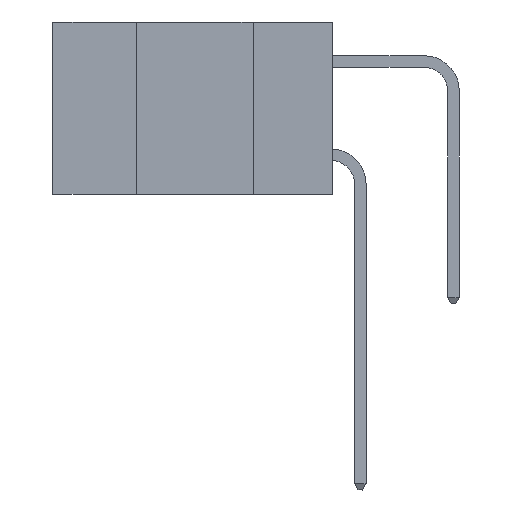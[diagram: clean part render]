
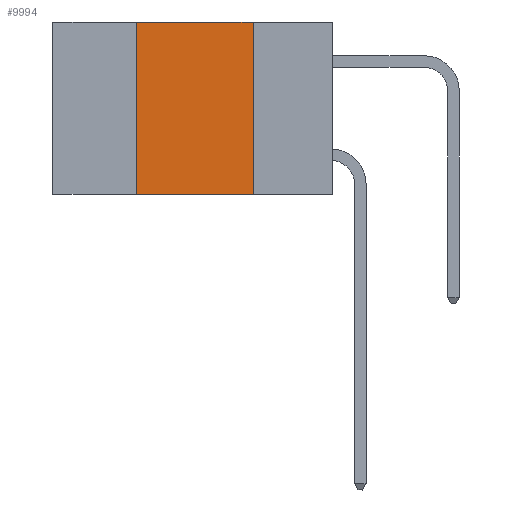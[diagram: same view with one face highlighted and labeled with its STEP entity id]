
A CAD part, left-side view. The second image highlights one B-rep face of the part: STEP entity #9994.
In plain terms, the highlighted planar face has unit normal (-1, 0, 0).
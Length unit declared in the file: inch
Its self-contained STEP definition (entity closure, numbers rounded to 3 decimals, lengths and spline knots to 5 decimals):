
#310 = CARTESIAN_POINT ( 'NONE',  ( 0., 0.42, 0. ) ) ;
#703 = FACE_OUTER_BOUND ( 'NONE', #6373, .T. ) ;
#1762 = LINE ( 'NONE', #10228, #7416 ) ;
#2990 = ORIENTED_EDGE ( 'NONE', *, *, #6395, .F. ) ;
#3064 = CARTESIAN_POINT ( 'NONE',  ( 0., 0.17, 0. ) ) ;
#3748 = LINE ( 'NONE', #3064, #11053 ) ;
#3896 = VERTEX_POINT ( 'NONE', #12928 ) ;
#4697 = DIRECTION ( 'NONE',  ( 0., 0., -1. ) ) ;
#4944 = VECTOR ( 'NONE', #11201, 39.37008 ) ;
#5253 = CARTESIAN_POINT ( 'NONE',  ( 0., 0.42, 0. ) ) ;
#5281 = DIRECTION ( 'NONE',  ( 0., -1., 0. ) ) ;
#5345 = CARTESIAN_POINT ( 'NONE',  ( 0., 0.6, 0. ) ) ;
#5495 = VERTEX_POINT ( 'NONE', #11802 ) ;
#6373 = EDGE_LOOP ( 'NONE', ( #9705, #7972, #2990, #8277 ) ) ;
#6395 = EDGE_CURVE ( 'NONE', #7828, #7204, #9927, .T. ) ;
#7115 = EDGE_CURVE ( 'NONE', #7828, #5495, #1762, .T. ) ;
#7204 = VERTEX_POINT ( 'NONE', #310 ) ;
#7416 = VECTOR ( 'NONE', #5281, 39.37008 ) ;
#7660 = CARTESIAN_POINT ( 'NONE',  ( 0., 0.6, 0. ) ) ;
#7828 = VERTEX_POINT ( 'NONE', #12256 ) ;
#7972 = ORIENTED_EDGE ( 'NONE', *, *, #8352, .F. ) ;
#8277 = ORIENTED_EDGE ( 'NONE', *, *, #7115, .T. ) ;
#8352 = EDGE_CURVE ( 'NONE', #7204, #3896, #9423, .T. ) ;
#9032 = DIRECTION ( 'NONE',  ( 0., 0., -1. ) ) ;
#9303 = AXIS2_PLACEMENT_3D ( 'NONE', #7660, #10658, #4697 ) ;
#9423 = LINE ( 'NONE', #5345, #10021 ) ;
#9705 = ORIENTED_EDGE ( 'NONE', *, *, #10878, .F. ) ;
#9927 = LINE ( 'NONE', #5253, #4944 ) ;
#9994 = ADVANCED_FACE ( 'NONE', ( #703 ), #12579, .F. ) ;
#10021 = VECTOR ( 'NONE', #11293, 39.37008 ) ;
#10228 = CARTESIAN_POINT ( 'NONE',  ( 0., 0.6, -0.37 ) ) ;
#10658 = DIRECTION ( 'NONE',  ( 1., 0., 0. ) ) ;
#10878 = EDGE_CURVE ( 'NONE', #3896, #5495, #3748, .T. ) ;
#11053 = VECTOR ( 'NONE', #9032, 39.37008 ) ;
#11201 = DIRECTION ( 'NONE',  ( 0., 0., 1. ) ) ;
#11293 = DIRECTION ( 'NONE',  ( 0., -1., 0. ) ) ;
#11802 = CARTESIAN_POINT ( 'NONE',  ( 0., 0.17, -0.37 ) ) ;
#12256 = CARTESIAN_POINT ( 'NONE',  ( 0., 0.42, -0.37 ) ) ;
#12579 = PLANE ( 'NONE',  #9303 ) ;
#12928 = CARTESIAN_POINT ( 'NONE',  ( 0., 0.17, 0. ) ) ;
